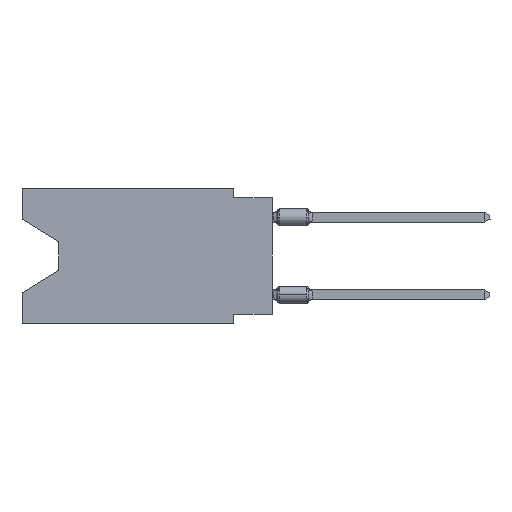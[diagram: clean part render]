
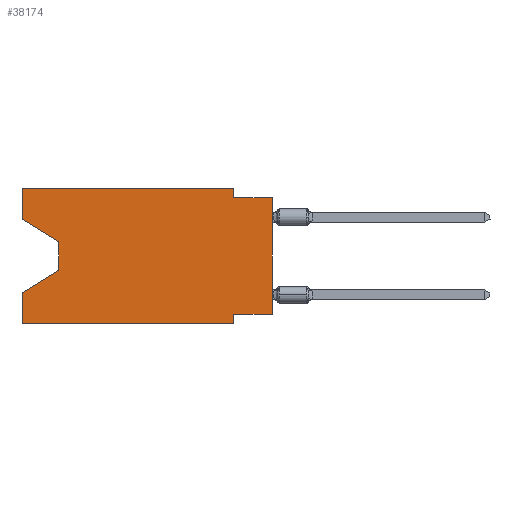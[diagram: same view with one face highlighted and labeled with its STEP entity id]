
A CAD part, left-side view. The second image highlights one B-rep face of the part: STEP entity #38174.
In plain terms, the highlighted planar face has unit normal (-1, 0, 0).
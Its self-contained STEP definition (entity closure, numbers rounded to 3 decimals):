
#192 = VECTOR ( 'NONE', #7488, 1000. ) ;
#193 = CARTESIAN_POINT ( 'NONE',  ( 0., 16.383, 0. ) ) ;
#1072 = CARTESIAN_POINT ( 'NONE',  ( 0., 16.383, 0. ) ) ;
#1375 = VERTEX_POINT ( 'NONE', #9507 ) ;
#1437 = CARTESIAN_POINT ( 'NONE',  ( 0., 2.54, -0.635 ) ) ;
#2164 = CARTESIAN_POINT ( 'NONE',  ( 0., 0., -0.635 ) ) ;
#2186 = VECTOR ( 'NONE', #29693, 1000. ) ;
#3036 = LINE ( 'NONE', #28568, #24154 ) ;
#3240 = DIRECTION ( 'NONE',  ( 0., 0., -1. ) ) ;
#3327 = LINE ( 'NONE', #32204, #38091 ) ;
#3491 = LINE ( 'NONE', #31545, #35448 ) ;
#3520 = VECTOR ( 'NONE', #18361, 1000. ) ;
#3943 = LINE ( 'NONE', #23808, #192 ) ;
#4116 = EDGE_LOOP ( 'NONE', ( #22311, #7556, #10694, #39954, #9879, #29360, #33026, #9119, #11678, #17024, #40749, #31479 ) ) ;
#4524 = LINE ( 'NONE', #2164, #27150 ) ;
#4673 = VECTOR ( 'NONE', #40356, 1000. ) ;
#4979 = LINE ( 'NONE', #36177, #2186 ) ;
#5565 = EDGE_CURVE ( 'NONE', #29524, #39162, #3327, .T. ) ;
#6687 = CARTESIAN_POINT ( 'NONE',  ( 0., 2.54, -8.89 ) ) ;
#7326 = EDGE_CURVE ( 'NONE', #34364, #22332, #3491, .T. ) ;
#7364 = CARTESIAN_POINT ( 'NONE',  ( 0., 16.383, 0. ) ) ;
#7488 = DIRECTION ( 'NONE',  ( 0., 0., 1. ) ) ;
#7556 = ORIENTED_EDGE ( 'NONE', *, *, #13878, .T. ) ;
#7755 = CARTESIAN_POINT ( 'NONE',  ( 0., 16.383, -6.852 ) ) ;
#8234 = EDGE_CURVE ( 'NONE', #16983, #39162, #4979, .T. ) ;
#8438 = CARTESIAN_POINT ( 'NONE',  ( 0., 13.97, -3.505 ) ) ;
#8485 = DIRECTION ( 'NONE',  ( 1., 0., 0. ) ) ;
#8993 = DIRECTION ( 'NONE',  ( 0., 0., -1. ) ) ;
#9119 = ORIENTED_EDGE ( 'NONE', *, *, #9168, .T. ) ;
#9168 = EDGE_CURVE ( 'NONE', #1375, #33713, #3943, .T. ) ;
#9507 = CARTESIAN_POINT ( 'NONE',  ( 0., 0., -8.255 ) ) ;
#9879 = ORIENTED_EDGE ( 'NONE', *, *, #32176, .T. ) ;
#10168 = CARTESIAN_POINT ( 'NONE',  ( 0., 2.54, 0. ) ) ;
#10469 = DIRECTION ( 'NONE',  ( 0., 1., 0. ) ) ;
#10669 = LINE ( 'NONE', #26780, #15707 ) ;
#10694 = ORIENTED_EDGE ( 'NONE', *, *, #8234, .T. ) ;
#11678 = ORIENTED_EDGE ( 'NONE', *, *, #12754, .F. ) ;
#12754 = EDGE_CURVE ( 'NONE', #27237, #33713, #4524, .T. ) ;
#13878 = EDGE_CURVE ( 'NONE', #22332, #16983, #33465, .T. ) ;
#14273 = AXIS2_PLACEMENT_3D ( 'NONE', #193, #8485, #8993 ) ;
#15707 = VECTOR ( 'NONE', #10469, 1000. ) ;
#16983 = VERTEX_POINT ( 'NONE', #38844 ) ;
#17024 = ORIENTED_EDGE ( 'NONE', *, *, #32856, .F. ) ;
#18361 = DIRECTION ( 'NONE',  ( 0., 0., -1. ) ) ;
#18830 = PLANE ( 'NONE',  #14273 ) ;
#18941 = DIRECTION ( 'NONE',  ( 0., -1., 0. ) ) ;
#20161 = DIRECTION ( 'NONE',  ( 0., -1., 0. ) ) ;
#20436 = DIRECTION ( 'NONE',  ( 0., -1., 0. ) ) ;
#21356 = VERTEX_POINT ( 'NONE', #1072 ) ;
#22252 = VECTOR ( 'NONE', #20161, 1000. ) ;
#22311 = ORIENTED_EDGE ( 'NONE', *, *, #7326, .T. ) ;
#22332 = VERTEX_POINT ( 'NONE', #8438 ) ;
#22481 = EDGE_CURVE ( 'NONE', #34364, #21356, #39175, .T. ) ;
#23808 = CARTESIAN_POINT ( 'NONE',  ( 0., 0., 0. ) ) ;
#24154 = VECTOR ( 'NONE', #18941, 1000. ) ;
#24612 = EDGE_CURVE ( 'NONE', #21356, #35864, #3036, .T. ) ;
#25305 = FACE_OUTER_BOUND ( 'NONE', #4116, .T. ) ;
#26019 = CARTESIAN_POINT ( 'NONE',  ( 0., 16.383, -8.89 ) ) ;
#26618 = DIRECTION ( 'NONE',  ( 0., 0., 1. ) ) ;
#26780 = CARTESIAN_POINT ( 'NONE',  ( 0., 0., -8.255 ) ) ;
#27150 = VECTOR ( 'NONE', #20436, 1000. ) ;
#27237 = VERTEX_POINT ( 'NONE', #1437 ) ;
#27769 = LINE ( 'NONE', #31327, #3520 ) ;
#28235 = EDGE_CURVE ( 'NONE', #1375, #29570, #10669, .T. ) ;
#28568 = CARTESIAN_POINT ( 'NONE',  ( 0., 16.383, 0. ) ) ;
#28569 = CARTESIAN_POINT ( 'NONE',  ( 0., 2.54, 0. ) ) ;
#28973 = VECTOR ( 'NONE', #3240, 1000. ) ;
#29062 = DIRECTION ( 'NONE',  ( 0., 0., 1. ) ) ;
#29360 = ORIENTED_EDGE ( 'NONE', *, *, #30525, .F. ) ;
#29524 = VERTEX_POINT ( 'NONE', #30384 ) ;
#29569 = LINE ( 'NONE', #26019, #22252 ) ;
#29570 = VERTEX_POINT ( 'NONE', #40215 ) ;
#29693 = DIRECTION ( 'NONE',  ( 0., 0.855, -0.519 ) ) ;
#30384 = CARTESIAN_POINT ( 'NONE',  ( 0., 16.383, -8.89 ) ) ;
#30523 = CARTESIAN_POINT ( 'NONE',  ( 0., 13.97, -3.505 ) ) ;
#30525 = EDGE_CURVE ( 'NONE', #29570, #32619, #27769, .T. ) ;
#31327 = CARTESIAN_POINT ( 'NONE',  ( 0., 2.54, -8.89 ) ) ;
#31479 = ORIENTED_EDGE ( 'NONE', *, *, #22481, .F. ) ;
#31545 = CARTESIAN_POINT ( 'NONE',  ( 0., 16.383, -2.038 ) ) ;
#31707 = LINE ( 'NONE', #28569, #28973 ) ;
#32021 = CARTESIAN_POINT ( 'NONE',  ( 0., 0., -0.635 ) ) ;
#32176 = EDGE_CURVE ( 'NONE', #29524, #32619, #29569, .T. ) ;
#32204 = CARTESIAN_POINT ( 'NONE',  ( 0., 16.383, 0. ) ) ;
#32619 = VERTEX_POINT ( 'NONE', #6687 ) ;
#32856 = EDGE_CURVE ( 'NONE', #35864, #27237, #31707, .T. ) ;
#33026 = ORIENTED_EDGE ( 'NONE', *, *, #28235, .F. ) ;
#33465 = LINE ( 'NONE', #30523, #4673 ) ;
#33713 = VERTEX_POINT ( 'NONE', #32021 ) ;
#33801 = CARTESIAN_POINT ( 'NONE',  ( 0., 16.383, -2.038 ) ) ;
#34364 = VERTEX_POINT ( 'NONE', #33801 ) ;
#35448 = VECTOR ( 'NONE', #38854, 1000. ) ;
#35864 = VERTEX_POINT ( 'NONE', #10168 ) ;
#36177 = CARTESIAN_POINT ( 'NONE',  ( 0., 13.97, -5.385 ) ) ;
#38091 = VECTOR ( 'NONE', #29062, 1000. ) ;
#38174 = ADVANCED_FACE ( 'NONE', ( #25305 ), #18830, .F. ) ;
#38844 = CARTESIAN_POINT ( 'NONE',  ( 0., 13.97, -5.385 ) ) ;
#38854 = DIRECTION ( 'NONE',  ( 0., -0.855, -0.519 ) ) ;
#39162 = VERTEX_POINT ( 'NONE', #7755 ) ;
#39175 = LINE ( 'NONE', #7364, #39357 ) ;
#39357 = VECTOR ( 'NONE', #26618, 1000. ) ;
#39954 = ORIENTED_EDGE ( 'NONE', *, *, #5565, .F. ) ;
#40215 = CARTESIAN_POINT ( 'NONE',  ( 0., 2.54, -8.255 ) ) ;
#40356 = DIRECTION ( 'NONE',  ( 0., 0., -1. ) ) ;
#40749 = ORIENTED_EDGE ( 'NONE', *, *, #24612, .F. ) ;
